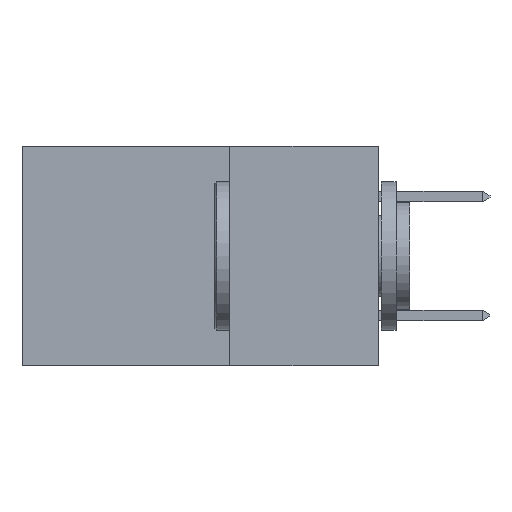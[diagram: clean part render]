
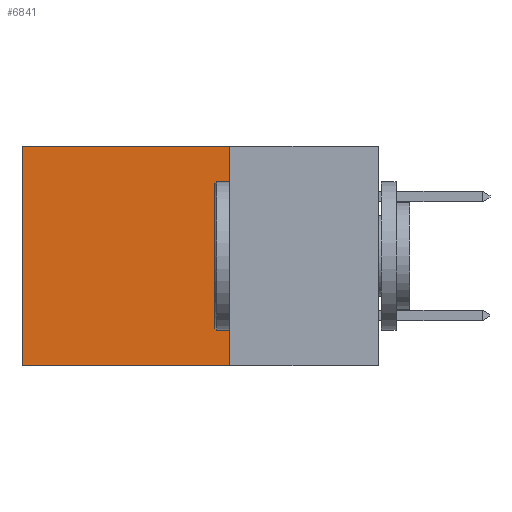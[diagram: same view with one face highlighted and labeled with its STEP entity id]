
A CAD part, left-side view. The second image highlights one B-rep face of the part: STEP entity #6841.
In plain terms, the highlighted planar face has unit normal (-1, 0, 0).
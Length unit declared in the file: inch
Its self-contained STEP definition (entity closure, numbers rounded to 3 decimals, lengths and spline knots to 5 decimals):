
#187 = AXIS2_PLACEMENT_3D ( 'NONE', #5399, #4492, #4588 ) ;
#552 = VECTOR ( 'NONE', #8743, 39.37008 ) ;
#583 = VECTOR ( 'NONE', #8906, 39.37008 ) ;
#1101 = LINE ( 'NONE', #8679, #552 ) ;
#1926 = CARTESIAN_POINT ( 'NONE',  ( 0.298, 0.25, -0.37 ) ) ;
#1932 = LINE ( 'NONE', #10045, #8558 ) ;
#2344 = LINE ( 'NONE', #4165, #583 ) ;
#2768 = DIRECTION ( 'NONE',  ( 0., 1., 0. ) ) ;
#2772 = VERTEX_POINT ( 'NONE', #5726 ) ;
#2844 = VERTEX_POINT ( 'NONE', #10540 ) ;
#2861 = ORIENTED_EDGE ( 'NONE', *, *, #7473, .F. ) ;
#3259 = EDGE_LOOP ( 'NONE', ( #7269, #9955, #2861, #7298 ) ) ;
#3306 = PLANE ( 'NONE',  #187 ) ;
#3961 = EDGE_CURVE ( 'NONE', #2844, #8654, #10277, .T. ) ;
#4165 = CARTESIAN_POINT ( 'NONE',  ( 0.298, 0.6, 0. ) ) ;
#4492 = DIRECTION ( 'NONE',  ( 1., 0., 0. ) ) ;
#4588 = DIRECTION ( 'NONE',  ( 0., 0., -1. ) ) ;
#5363 = FACE_OUTER_BOUND ( 'NONE', #3259, .T. ) ;
#5399 = CARTESIAN_POINT ( 'NONE',  ( 0.298, 0.25, 0. ) ) ;
#5454 = CARTESIAN_POINT ( 'NONE',  ( 0.298, 0.6, 0. ) ) ;
#5726 = CARTESIAN_POINT ( 'NONE',  ( 0.298, 0.25, 0. ) ) ;
#5829 = EDGE_CURVE ( 'NONE', #9788, #8654, #2344, .T. ) ;
#5880 = CARTESIAN_POINT ( 'NONE',  ( 0.298, 0.6, -0.37 ) ) ;
#6628 = VECTOR ( 'NONE', #2768, 39.37008 ) ;
#6841 = ADVANCED_FACE ( 'NONE', ( #5363 ), #3306, .F. ) ;
#7269 = ORIENTED_EDGE ( 'NONE', *, *, #5829, .T. ) ;
#7298 = ORIENTED_EDGE ( 'NONE', *, *, #9034, .T. ) ;
#7473 = EDGE_CURVE ( 'NONE', #2772, #2844, #1101, .T. ) ;
#8558 = VECTOR ( 'NONE', #9243, 39.37008 ) ;
#8654 = VERTEX_POINT ( 'NONE', #5880 ) ;
#8679 = CARTESIAN_POINT ( 'NONE',  ( 0.298, 0.25, 0. ) ) ;
#8743 = DIRECTION ( 'NONE',  ( 0., 0., -1. ) ) ;
#8906 = DIRECTION ( 'NONE',  ( 0., 0., -1. ) ) ;
#9034 = EDGE_CURVE ( 'NONE', #2772, #9788, #1932, .T. ) ;
#9243 = DIRECTION ( 'NONE',  ( 0., 1., 0. ) ) ;
#9788 = VERTEX_POINT ( 'NONE', #5454 ) ;
#9955 = ORIENTED_EDGE ( 'NONE', *, *, #3961, .F. ) ;
#10045 = CARTESIAN_POINT ( 'NONE',  ( 0.298, 0.25, 0. ) ) ;
#10277 = LINE ( 'NONE', #1926, #6628 ) ;
#10540 = CARTESIAN_POINT ( 'NONE',  ( 0.298, 0.25, -0.37 ) ) ;
